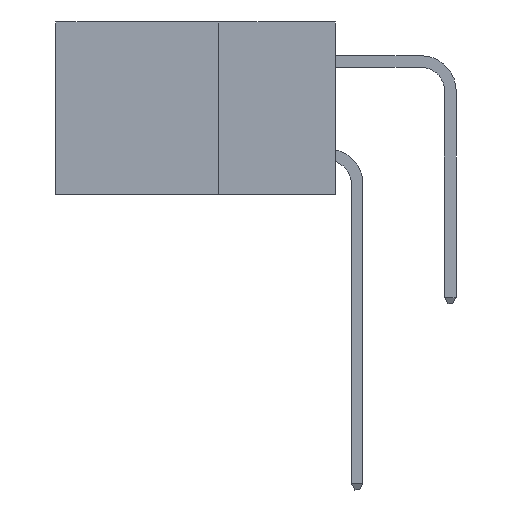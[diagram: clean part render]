
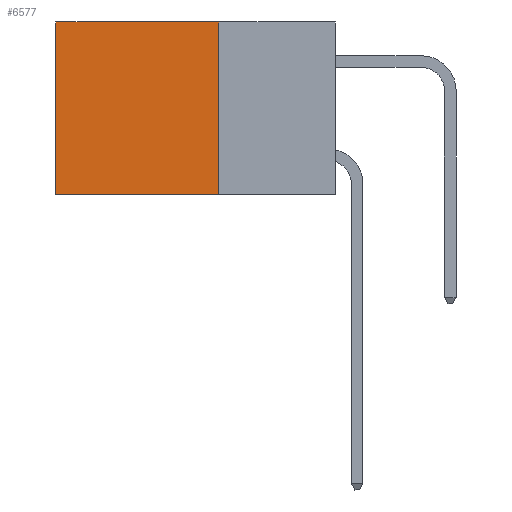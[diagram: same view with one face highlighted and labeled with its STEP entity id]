
A CAD part, left-side view. The second image highlights one B-rep face of the part: STEP entity #6577.
In plain terms, the highlighted planar face has unit normal (-1, 0, 0).
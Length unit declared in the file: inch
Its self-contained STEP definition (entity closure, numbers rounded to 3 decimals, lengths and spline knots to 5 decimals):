
#794 = VERTEX_POINT ( 'NONE', #9336 ) ;
#1252 = LINE ( 'NONE', #24291, #20146 ) ;
#1596 = DIRECTION ( 'NONE',  ( 0., 1., 0. ) ) ;
#3132 = DIRECTION ( 'NONE',  ( 0., 0., -1. ) ) ;
#3747 = DIRECTION ( 'NONE',  ( 0., 0., -1. ) ) ;
#6561 = ORIENTED_EDGE ( 'NONE', *, *, #29501, .T. ) ;
#6577 = ADVANCED_FACE ( 'NONE', ( #26529 ), #21346, .F. ) ;
#6693 = ORIENTED_EDGE ( 'NONE', *, *, #24662, .F. ) ;
#7182 = CARTESIAN_POINT ( 'NONE',  ( 0.2875, 0.25, 0. ) ) ;
#8011 = EDGE_CURVE ( 'NONE', #21884, #794, #16011, .T. ) ;
#9336 = CARTESIAN_POINT ( 'NONE',  ( 0.2875, 0.6, -0.37 ) ) ;
#11089 = ORIENTED_EDGE ( 'NONE', *, *, #20779, .T. ) ;
#16011 = LINE ( 'NONE', #21529, #35695 ) ;
#16586 = VERTEX_POINT ( 'NONE', #20217 ) ;
#19204 = CARTESIAN_POINT ( 'NONE',  ( 0.2875, 0.25, 0. ) ) ;
#20146 = VECTOR ( 'NONE', #3132, 39.37008 ) ;
#20217 = CARTESIAN_POINT ( 'NONE',  ( 0.2875, 0.25, 0. ) ) ;
#20479 = LINE ( 'NONE', #43713, #37957 ) ;
#20779 = EDGE_CURVE ( 'NONE', #22211, #794, #1252, .T. ) ;
#21346 = PLANE ( 'NONE',  #32237 ) ;
#21529 = CARTESIAN_POINT ( 'NONE',  ( 0.2875, 0.25, -0.37 ) ) ;
#21884 = VERTEX_POINT ( 'NONE', #22852 ) ;
#22211 = VERTEX_POINT ( 'NONE', #27949 ) ;
#22708 = DIRECTION ( 'NONE',  ( 0., 0., -1. ) ) ;
#22852 = CARTESIAN_POINT ( 'NONE',  ( 0.2875, 0.25, -0.37 ) ) ;
#24291 = CARTESIAN_POINT ( 'NONE',  ( 0.2875, 0.6, 0. ) ) ;
#24662 = EDGE_CURVE ( 'NONE', #16586, #21884, #34000, .T. ) ;
#24852 = DIRECTION ( 'NONE',  ( 1., 0., 0. ) ) ;
#26529 = FACE_OUTER_BOUND ( 'NONE', #39877, .T. ) ;
#27949 = CARTESIAN_POINT ( 'NONE',  ( 0.2875, 0.6, 0. ) ) ;
#29501 = EDGE_CURVE ( 'NONE', #16586, #22211, #20479, .T. ) ;
#32061 = DIRECTION ( 'NONE',  ( 0., 1., 0. ) ) ;
#32237 = AXIS2_PLACEMENT_3D ( 'NONE', #7182, #24852, #3747 ) ;
#32898 = VECTOR ( 'NONE', #22708, 39.37008 ) ;
#34000 = LINE ( 'NONE', #19204, #32898 ) ;
#35695 = VECTOR ( 'NONE', #32061, 39.37008 ) ;
#36225 = ORIENTED_EDGE ( 'NONE', *, *, #8011, .F. ) ;
#37957 = VECTOR ( 'NONE', #1596, 39.37008 ) ;
#39877 = EDGE_LOOP ( 'NONE', ( #11089, #36225, #6693, #6561 ) ) ;
#43713 = CARTESIAN_POINT ( 'NONE',  ( 0.2875, 0.25, 0. ) ) ;
